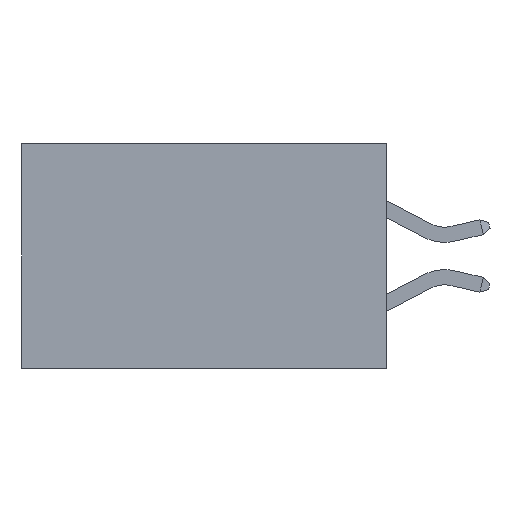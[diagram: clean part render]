
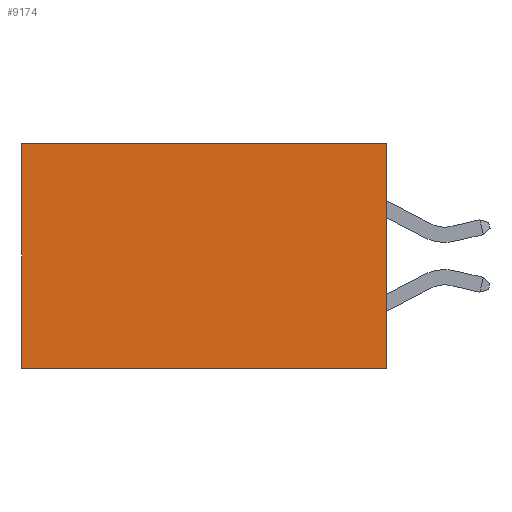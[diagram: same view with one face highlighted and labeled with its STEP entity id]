
A CAD part, left-side view. The second image highlights one B-rep face of the part: STEP entity #9174.
In plain terms, the highlighted planar face has unit normal (-1, 0, 0).
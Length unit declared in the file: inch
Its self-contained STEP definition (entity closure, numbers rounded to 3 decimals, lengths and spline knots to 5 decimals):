
#252 = PLANE ( 'NONE',  #10846 ) ;
#764 = CARTESIAN_POINT ( 'NONE',  ( 0.298, 0., 0. ) ) ;
#1148 = DIRECTION ( 'NONE',  ( 1., 0., 0. ) ) ;
#1247 = CARTESIAN_POINT ( 'NONE',  ( 0.298, 0., 0. ) ) ;
#1885 = LINE ( 'NONE', #764, #9888 ) ;
#2027 = CARTESIAN_POINT ( 'NONE',  ( 0.298, 0.6, 0. ) ) ;
#2147 = CARTESIAN_POINT ( 'NONE',  ( 0.298, 0., -0.37 ) ) ;
#2689 = ORIENTED_EDGE ( 'NONE', *, *, #5158, .F. ) ;
#3391 = VECTOR ( 'NONE', #3936, 39.37008 ) ;
#3920 = DIRECTION ( 'NONE',  ( 0., 0., -1. ) ) ;
#3936 = DIRECTION ( 'NONE',  ( 0., 0., -1. ) ) ;
#4591 = EDGE_CURVE ( 'NONE', #11589, #4704, #7355, .T. ) ;
#4673 = VERTEX_POINT ( 'NONE', #6638 ) ;
#4700 = DIRECTION ( 'NONE',  ( 0., 0., -1. ) ) ;
#4704 = VERTEX_POINT ( 'NONE', #2147 ) ;
#4789 = ORIENTED_EDGE ( 'NONE', *, *, #7520, .T. ) ;
#4796 = DIRECTION ( 'NONE',  ( 0., 1., 0. ) ) ;
#4985 = EDGE_LOOP ( 'NONE', ( #5194, #2689, #5383, #4789 ) ) ;
#5158 = EDGE_CURVE ( 'NONE', #4704, #10763, #9352, .T. ) ;
#5194 = ORIENTED_EDGE ( 'NONE', *, *, #6377, .T. ) ;
#5383 = ORIENTED_EDGE ( 'NONE', *, *, #4591, .F. ) ;
#6337 = VECTOR ( 'NONE', #4700, 39.37008 ) ;
#6377 = EDGE_CURVE ( 'NONE', #4673, #10763, #11476, .T. ) ;
#6468 = CARTESIAN_POINT ( 'NONE',  ( 0.298, 0., 0. ) ) ;
#6638 = CARTESIAN_POINT ( 'NONE',  ( 0.298, 0.6, 0. ) ) ;
#7355 = LINE ( 'NONE', #1247, #3391 ) ;
#7520 = EDGE_CURVE ( 'NONE', #11589, #4673, #1885, .T. ) ;
#8642 = VECTOR ( 'NONE', #4796, 39.37008 ) ;
#9174 = ADVANCED_FACE ( 'NONE', ( #10601 ), #252, .F. ) ;
#9352 = LINE ( 'NONE', #10271, #8642 ) ;
#9888 = VECTOR ( 'NONE', #10027, 39.37008 ) ;
#10009 = CARTESIAN_POINT ( 'NONE',  ( 0.298, 0.6, -0.37 ) ) ;
#10027 = DIRECTION ( 'NONE',  ( 0., 1., 0. ) ) ;
#10271 = CARTESIAN_POINT ( 'NONE',  ( 0.298, 0., -0.37 ) ) ;
#10601 = FACE_OUTER_BOUND ( 'NONE', #4985, .T. ) ;
#10763 = VERTEX_POINT ( 'NONE', #10009 ) ;
#10846 = AXIS2_PLACEMENT_3D ( 'NONE', #11258, #1148, #3920 ) ;
#11258 = CARTESIAN_POINT ( 'NONE',  ( 0.298, 0., 0. ) ) ;
#11476 = LINE ( 'NONE', #2027, #6337 ) ;
#11589 = VERTEX_POINT ( 'NONE', #6468 ) ;
